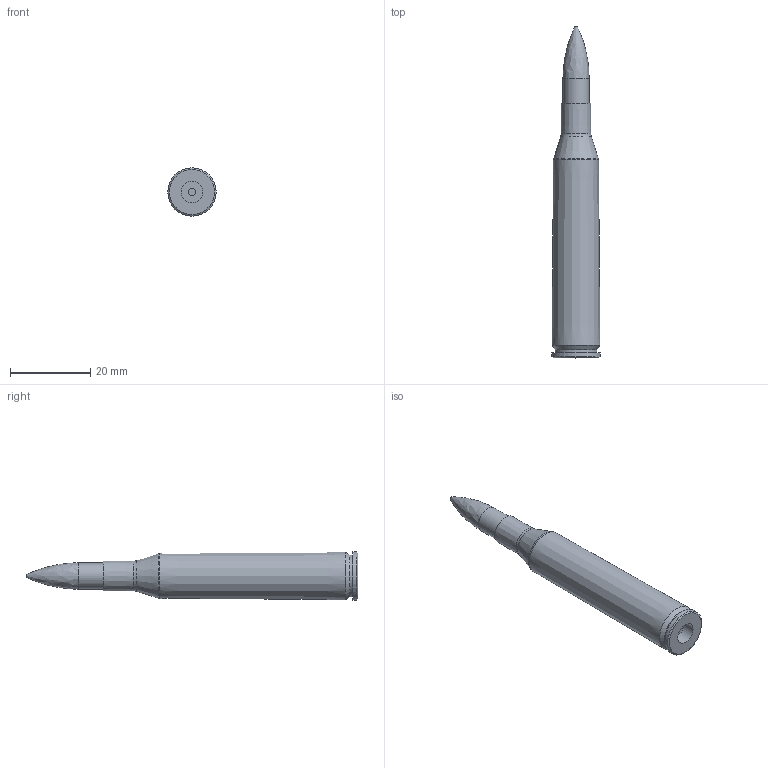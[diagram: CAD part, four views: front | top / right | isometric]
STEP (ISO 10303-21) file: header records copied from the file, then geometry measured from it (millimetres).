
FILE_DESCRIPTION((''),'2;1');
FILE_NAME('25-06 Remington.stp','2013-02-20T13:04:51',('agarrett'),(''),'Autodesk Inventor 2012','Autodesk Inventor 2012','');
FILE_SCHEMA(('AUTOMOTIVE_DESIGN { 1 0 10303 214 1 1 1 1 }'));
Length unit declared in the file: inch
Products named in the file (3): Rimless Bottleneck Assembly; Rimless Bottleneck; SpitzerPoint
Assembly tree (2 placements, depth 2):
  Rimless Bottleneck Assembly
    Rimless Bottleneck
    SpitzerPoint
Bounding box: 12.01 x 82.55 x 12.01 mm (x, y, z)
Volume: 2280.8 mm3; surface area: 5101.8 mm2
Topology: 2 solids, 2 shells, 27 faces, 46 edges, 26 vertices
Faces by surface type: cone 8, torus 6, plane 6, cylinder 5, bspline 1, sphere 1
Full cylindrical faces by diameter (mm): 1.778 x1, 5.334 x1, 6.541 x1, 10.389 x1, 12.014 x1
Entity records: 655 total; most frequent: DIRECTION 114, CARTESIAN_POINT 110, AXIS2_PLACEMENT_3D 57, ORIENTED_EDGE 52, EDGE_LOOP 52, FACE_OUTER_BOUND 27, ADVANCED_FACE 27, VERTEX_POINT 26
